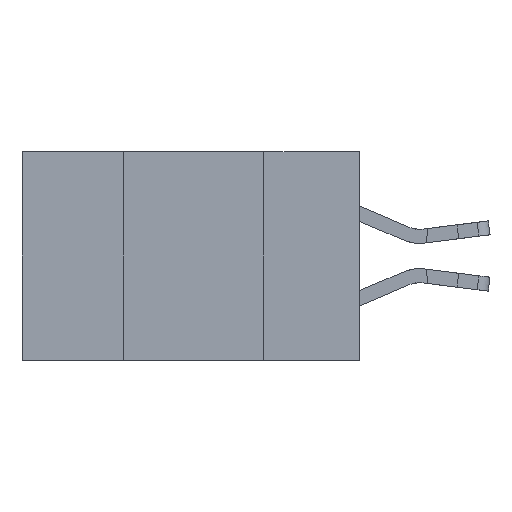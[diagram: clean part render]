
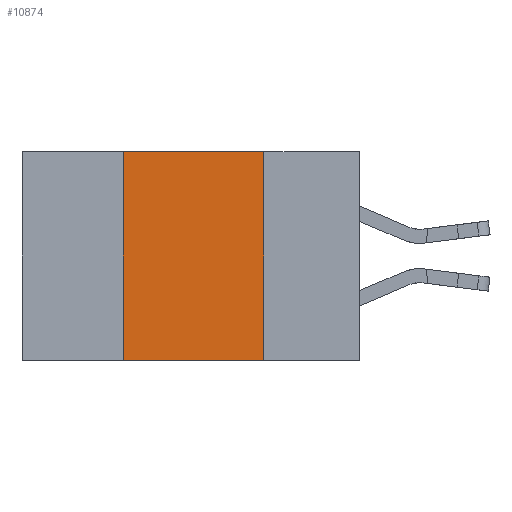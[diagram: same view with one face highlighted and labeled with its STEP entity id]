
A CAD part, left-side view. The second image highlights one B-rep face of the part: STEP entity #10874.
In plain terms, the highlighted planar face has unit normal (-1, 0, 0).
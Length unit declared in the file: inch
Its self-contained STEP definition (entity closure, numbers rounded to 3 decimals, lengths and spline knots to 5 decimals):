
#1843 = LINE ( 'NONE', #10206, #15397 ) ;
#2062 = CARTESIAN_POINT ( 'NONE',  ( 0., 0.17, -0.37 ) ) ;
#2855 = ORIENTED_EDGE ( 'NONE', *, *, #7331, .F. ) ;
#4466 = EDGE_CURVE ( 'NONE', #16759, #10325, #10627, .T. ) ;
#5472 = ORIENTED_EDGE ( 'NONE', *, *, #23060, .F. ) ;
#6411 = VECTOR ( 'NONE', #19258, 39.37008 ) ;
#6966 = CARTESIAN_POINT ( 'NONE',  ( 0., 0.6, 0. ) ) ;
#7240 = CARTESIAN_POINT ( 'NONE',  ( 0., 0.42, 0. ) ) ;
#7331 = EDGE_CURVE ( 'NONE', #10325, #15374, #1843, .T. ) ;
#7344 = CARTESIAN_POINT ( 'NONE',  ( 0., 0.6, -0.37 ) ) ;
#7356 = ORIENTED_EDGE ( 'NONE', *, *, #16274, .T. ) ;
#7360 = AXIS2_PLACEMENT_3D ( 'NONE', #6966, #9024, #15045 ) ;
#9024 = DIRECTION ( 'NONE',  ( 1., 0., 0. ) ) ;
#9486 = DIRECTION ( 'NONE',  ( 0., 0., 1. ) ) ;
#9652 = CARTESIAN_POINT ( 'NONE',  ( 0., 0.6, 0. ) ) ;
#9805 = CARTESIAN_POINT ( 'NONE',  ( 0., 0.42, 0. ) ) ;
#10040 = FACE_OUTER_BOUND ( 'NONE', #17204, .T. ) ;
#10206 = CARTESIAN_POINT ( 'NONE',  ( 0., 0.17, 0. ) ) ;
#10325 = VERTEX_POINT ( 'NONE', #20476 ) ;
#10627 = LINE ( 'NONE', #9652, #18733 ) ;
#10874 = ADVANCED_FACE ( 'NONE', ( #10040 ), #16840, .F. ) ;
#14851 = VECTOR ( 'NONE', #9486, 39.37008 ) ;
#15045 = DIRECTION ( 'NONE',  ( 0., 0., -1. ) ) ;
#15374 = VERTEX_POINT ( 'NONE', #2062 ) ;
#15397 = VECTOR ( 'NONE', #16107, 39.37008 ) ;
#16107 = DIRECTION ( 'NONE',  ( 0., 0., -1. ) ) ;
#16274 = EDGE_CURVE ( 'NONE', #21387, #15374, #17849, .T. ) ;
#16759 = VERTEX_POINT ( 'NONE', #9805 ) ;
#16840 = PLANE ( 'NONE',  #7360 ) ;
#17204 = EDGE_LOOP ( 'NONE', ( #2855, #21048, #5472, #7356 ) ) ;
#17378 = DIRECTION ( 'NONE',  ( 0., -1., 0. ) ) ;
#17849 = LINE ( 'NONE', #7344, #6411 ) ;
#18733 = VECTOR ( 'NONE', #17378, 39.37008 ) ;
#19258 = DIRECTION ( 'NONE',  ( 0., -1., 0. ) ) ;
#20476 = CARTESIAN_POINT ( 'NONE',  ( 0., 0.17, 0. ) ) ;
#21048 = ORIENTED_EDGE ( 'NONE', *, *, #4466, .F. ) ;
#21387 = VERTEX_POINT ( 'NONE', #24819 ) ;
#23060 = EDGE_CURVE ( 'NONE', #21387, #16759, #24848, .T. ) ;
#24819 = CARTESIAN_POINT ( 'NONE',  ( 0., 0.42, -0.37 ) ) ;
#24848 = LINE ( 'NONE', #7240, #14851 ) ;
